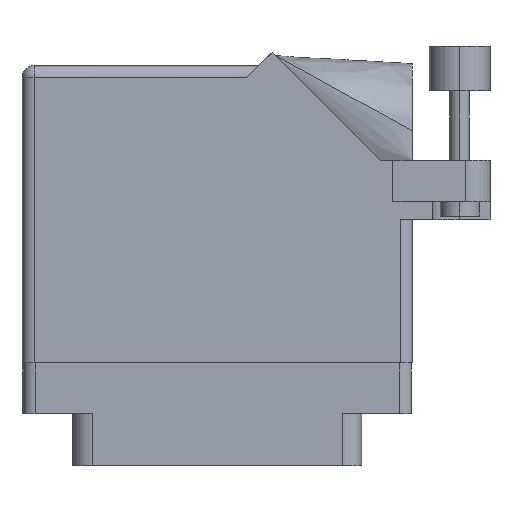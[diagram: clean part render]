
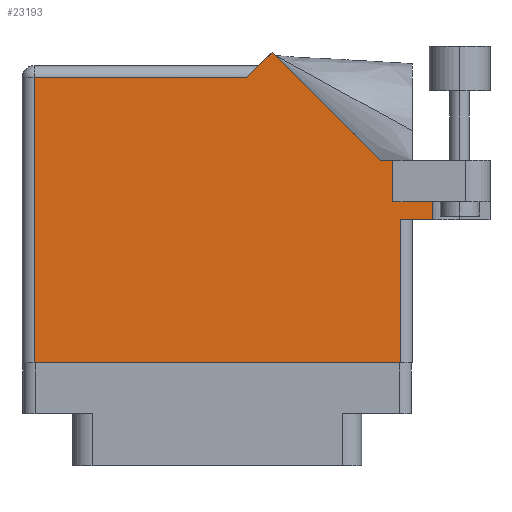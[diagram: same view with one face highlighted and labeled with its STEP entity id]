
A CAD part, front view. The second image highlights one B-rep face of the part: STEP entity #23193.
In plain terms, the highlighted face is planar.
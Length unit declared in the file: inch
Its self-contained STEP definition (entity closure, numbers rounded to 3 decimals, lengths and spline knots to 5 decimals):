
#530 = CARTESIAN_POINT ( 'NONE',  ( 0., 0., 0. ) ) ;
#3460 = CARTESIAN_POINT ( 'NONE',  ( 1.217, 1.53, 0. ) ) ;
#3559 = ORIENTED_EDGE ( 'NONE', *, *, #13052, .T. ) ;
#4207 = LINE ( 'NONE', #31659, #23721 ) ;
#4290 = VERTEX_POINT ( 'NONE', #14815 ) ;
#4424 = VERTEX_POINT ( 'NONE', #27540 ) ;
#4478 = VERTEX_POINT ( 'NONE', #23086 ) ;
#4819 = ORIENTED_EDGE ( 'NONE', *, *, #5246, .F. ) ;
#5134 = VECTOR ( 'NONE', #22172, 39.37008 ) ;
#5246 = EDGE_CURVE ( 'NONE', #4424, #7505, #25011, .T. ) ;
#5419 = CARTESIAN_POINT ( 'NONE',  ( 0., 1.468, 0. ) ) ;
#5531 = LINE ( 'NONE', #530, #32768 ) ;
#5597 = ORIENTED_EDGE ( 'NONE', *, *, #26154, .T. ) ;
#5709 = DIRECTION ( 'NONE',  ( 1., 0., 0. ) ) ;
#6031 = DIRECTION ( 'NONE',  ( 0., 1., 0. ) ) ;
#6237 = LINE ( 'NONE', #3460, #9702 ) ;
#6368 = EDGE_CURVE ( 'NONE', #7505, #36959, #23440, .T. ) ;
#6434 = CARTESIAN_POINT ( 'NONE',  ( 1.91, 0.831, 0. ) ) ;
#6629 = DIRECTION ( 'NONE',  ( -0.707, -0.707, 0. ) ) ;
#6766 = CARTESIAN_POINT ( 'NONE',  ( 1.948, 0.737, 0. ) ) ;
#7313 = EDGE_CURVE ( 'NONE', #4478, #10197, #11588, .T. ) ;
#7416 = CARTESIAN_POINT ( 'NONE',  ( 2.1115, 0.831, 0. ) ) ;
#7505 = VERTEX_POINT ( 'NONE', #7416 ) ;
#8537 = DIRECTION ( 'NONE',  ( -0.707, 0.707, 0. ) ) ;
#8764 = PLANE ( 'NONE',  #34863 ) ;
#9611 = LINE ( 'NONE', #35761, #33064 ) ;
#9702 = VECTOR ( 'NONE', #6629, 39.37008 ) ;
#10197 = VERTEX_POINT ( 'NONE', #6766 ) ;
#10786 = VECTOR ( 'NONE', #20426, 39.37008 ) ;
#11568 = DIRECTION ( 'NONE',  ( -1., 0., 0. ) ) ;
#11588 = LINE ( 'NONE', #23745, #38827 ) ;
#12007 = LINE ( 'NONE', #6434, #33925 ) ;
#12289 = EDGE_CURVE ( 'NONE', #37955, #26498, #25313, .T. ) ;
#12511 = FACE_OUTER_BOUND ( 'NONE', #34616, .T. ) ;
#12772 = VERTEX_POINT ( 'NONE', #20978 ) ;
#12940 = CARTESIAN_POINT ( 'NONE',  ( 1.155, 1.468, 0. ) ) ;
#13052 = EDGE_CURVE ( 'NONE', #10197, #36959, #21982, .T. ) ;
#13356 = CARTESIAN_POINT ( 'NONE',  ( 1.84442, 1.044, 0. ) ) ;
#14209 = CARTESIAN_POINT ( 'NONE',  ( 1.84442, 1.044, 0. ) ) ;
#14815 = CARTESIAN_POINT ( 'NONE',  ( 1.91, 1.044, 0. ) ) ;
#15192 = EDGE_CURVE ( 'NONE', #26498, #17926, #6237, .T. ) ;
#15526 = ORIENTED_EDGE ( 'NONE', *, *, #25866, .T. ) ;
#16333 = DIRECTION ( 'NONE',  ( -1., 0., 0. ) ) ;
#16515 = VECTOR ( 'NONE', #8537, 39.37008 ) ;
#17198 = DIRECTION ( 'NONE',  ( 0., 0., -1. ) ) ;
#17726 = ORIENTED_EDGE ( 'NONE', *, *, #6368, .F. ) ;
#17926 = VERTEX_POINT ( 'NONE', #12940 ) ;
#20426 = DIRECTION ( 'NONE',  ( 0., -1., 0. ) ) ;
#20908 = LINE ( 'NONE', #5419, #24370 ) ;
#20978 = CARTESIAN_POINT ( 'NONE',  ( 0.062, 0., 0. ) ) ;
#21615 = DIRECTION ( 'NONE',  ( 1., 0., 0. ) ) ;
#21744 = DIRECTION ( 'NONE',  ( 0., -1., 0. ) ) ;
#21982 = LINE ( 'NONE', #34524, #5134 ) ;
#22172 = DIRECTION ( 'NONE',  ( 1., 0., 0. ) ) ;
#22662 = CARTESIAN_POINT ( 'NONE',  ( 2.1115, 1.16177, 0. ) ) ;
#22690 = CARTESIAN_POINT ( 'NONE',  ( 1.28771, 1.60071, 0. ) ) ;
#23086 = CARTESIAN_POINT ( 'NONE',  ( 1.948, 0., 0. ) ) ;
#23193 = ADVANCED_FACE ( 'NONE', ( #12511 ), #8764, .F. ) ;
#23440 = LINE ( 'NONE', #22662, #10786 ) ;
#23721 = VECTOR ( 'NONE', #16333, 39.37008 ) ;
#23745 = CARTESIAN_POINT ( 'NONE',  ( 1.948, 0.737, 0. ) ) ;
#24370 = VECTOR ( 'NONE', #11568, 39.37008 ) ;
#24841 = DIRECTION ( 'NONE',  ( -1., 0., 0. ) ) ;
#25011 = LINE ( 'NONE', #28561, #25660 ) ;
#25202 = CARTESIAN_POINT ( 'NONE',  ( 0.062, 1.468, 0. ) ) ;
#25277 = EDGE_CURVE ( 'NONE', #4290, #37955, #4207, .T. ) ;
#25313 = LINE ( 'NONE', #13356, #16515 ) ;
#25660 = VECTOR ( 'NONE', #21615, 39.37008 ) ;
#25866 = EDGE_CURVE ( 'NONE', #4424, #4290, #12007, .T. ) ;
#26154 = EDGE_CURVE ( 'NONE', #17926, #27915, #20908, .T. ) ;
#26498 = VERTEX_POINT ( 'NONE', #22690 ) ;
#27082 = ORIENTED_EDGE ( 'NONE', *, *, #31252, .T. ) ;
#27540 = CARTESIAN_POINT ( 'NONE',  ( 1.91, 0.831, 0. ) ) ;
#27737 = EDGE_CURVE ( 'NONE', #12772, #4478, #5531, .T. ) ;
#27915 = VERTEX_POINT ( 'NONE', #25202 ) ;
#28561 = CARTESIAN_POINT ( 'NONE',  ( 1.91, 0.831, 0. ) ) ;
#30330 = DIRECTION ( 'NONE',  ( 0., 1., 0. ) ) ;
#31252 = EDGE_CURVE ( 'NONE', #27915, #12772, #9611, .T. ) ;
#31475 = CARTESIAN_POINT ( 'NONE',  ( 2.1115, 0.737, 0. ) ) ;
#31659 = CARTESIAN_POINT ( 'NONE',  ( 2.41, 1.044, 0. ) ) ;
#31684 = ORIENTED_EDGE ( 'NONE', *, *, #12289, .T. ) ;
#32768 = VECTOR ( 'NONE', #5709, 39.37008 ) ;
#32962 = ORIENTED_EDGE ( 'NONE', *, *, #25277, .T. ) ;
#33064 = VECTOR ( 'NONE', #21744, 39.37008 ) ;
#33828 = ORIENTED_EDGE ( 'NONE', *, *, #15192, .T. ) ;
#33925 = VECTOR ( 'NONE', #30330, 39.37008 ) ;
#34284 = ORIENTED_EDGE ( 'NONE', *, *, #27737, .T. ) ;
#34398 = CARTESIAN_POINT ( 'NONE',  ( 0., 1.53, 0. ) ) ;
#34524 = CARTESIAN_POINT ( 'NONE',  ( 2.01, 0.737, 0. ) ) ;
#34616 = EDGE_LOOP ( 'NONE', ( #34284, #36213, #3559, #17726, #4819, #15526, #32962, #31684, #33828, #5597, #27082 ) ) ;
#34863 = AXIS2_PLACEMENT_3D ( 'NONE', #34398, #17198, #24841 ) ;
#35761 = CARTESIAN_POINT ( 'NONE',  ( 0.062, 0., 0. ) ) ;
#36213 = ORIENTED_EDGE ( 'NONE', *, *, #7313, .T. ) ;
#36959 = VERTEX_POINT ( 'NONE', #31475 ) ;
#37955 = VERTEX_POINT ( 'NONE', #14209 ) ;
#38827 = VECTOR ( 'NONE', #6031, 39.37008 ) ;
